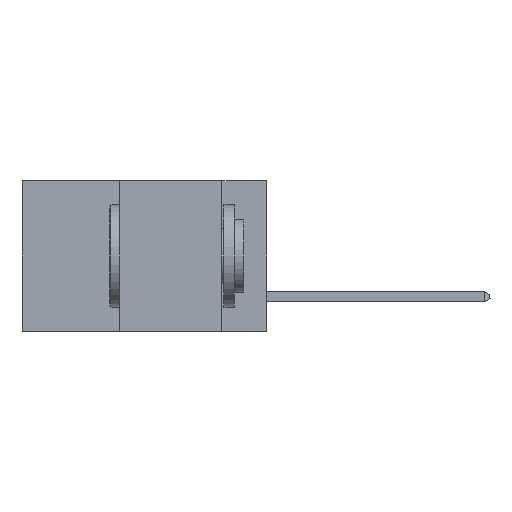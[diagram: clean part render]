
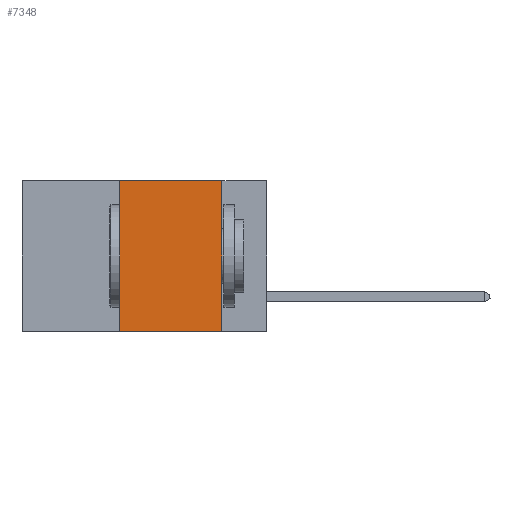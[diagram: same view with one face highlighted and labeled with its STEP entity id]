
A CAD part, left-side view. The second image highlights one B-rep face of the part: STEP entity #7348.
In plain terms, the highlighted planar face has unit normal (-1, 0, 0).
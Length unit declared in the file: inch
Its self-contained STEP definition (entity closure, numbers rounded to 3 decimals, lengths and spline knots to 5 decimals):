
#431 = PLANE ( 'NONE',  #6124 ) ;
#549 = CARTESIAN_POINT ( 'NONE',  ( 0., 0.11, 0. ) ) ;
#1457 = LINE ( 'NONE', #8923, #3112 ) ;
#1663 = EDGE_CURVE ( 'NONE', #2905, #11266, #1457, .T. ) ;
#2905 = VERTEX_POINT ( 'NONE', #17620 ) ;
#3067 = DIRECTION ( 'NONE',  ( 0., -1., 0. ) ) ;
#3112 = VECTOR ( 'NONE', #10930, 39.37008 ) ;
#3294 = ORIENTED_EDGE ( 'NONE', *, *, #11634, .F. ) ;
#3508 = DIRECTION ( 'NONE',  ( 1., 0., 0. ) ) ;
#3814 = VECTOR ( 'NONE', #6072, 39.37008 ) ;
#3959 = ORIENTED_EDGE ( 'NONE', *, *, #1663, .F. ) ;
#4521 = CARTESIAN_POINT ( 'NONE',  ( 0., 0.6, -0.37 ) ) ;
#4826 = DIRECTION ( 'NONE',  ( 0., 0., -1. ) ) ;
#5379 = FACE_OUTER_BOUND ( 'NONE', #9659, .T. ) ;
#5426 = VECTOR ( 'NONE', #3067, 39.37008 ) ;
#6072 = DIRECTION ( 'NONE',  ( 0., 0., -1. ) ) ;
#6124 = AXIS2_PLACEMENT_3D ( 'NONE', #12545, #3508, #4826 ) ;
#6180 = ORIENTED_EDGE ( 'NONE', *, *, #19208, .T. ) ;
#7348 = ADVANCED_FACE ( 'NONE', ( #5379 ), #431, .F. ) ;
#7781 = LINE ( 'NONE', #17904, #3814 ) ;
#8299 = VERTEX_POINT ( 'NONE', #9223 ) ;
#8686 = CARTESIAN_POINT ( 'NONE',  ( 0., 0.11, -0.37 ) ) ;
#8923 = CARTESIAN_POINT ( 'NONE',  ( 0., 0.6, 0. ) ) ;
#9223 = CARTESIAN_POINT ( 'NONE',  ( 0., 0.36, -0.37 ) ) ;
#9659 = EDGE_LOOP ( 'NONE', ( #9702, #3959, #3294, #6180 ) ) ;
#9702 = ORIENTED_EDGE ( 'NONE', *, *, #13621, .F. ) ;
#10371 = VERTEX_POINT ( 'NONE', #8686 ) ;
#10930 = DIRECTION ( 'NONE',  ( 0., -1., 0. ) ) ;
#11266 = VERTEX_POINT ( 'NONE', #549 ) ;
#11634 = EDGE_CURVE ( 'NONE', #8299, #2905, #18638, .T. ) ;
#11795 = DIRECTION ( 'NONE',  ( 0., 0., 1. ) ) ;
#12545 = CARTESIAN_POINT ( 'NONE',  ( 0., 0.6, 0. ) ) ;
#13621 = EDGE_CURVE ( 'NONE', #11266, #10371, #7781, .T. ) ;
#14674 = CARTESIAN_POINT ( 'NONE',  ( 0., 0.36, 0. ) ) ;
#15308 = VECTOR ( 'NONE', #11795, 39.37008 ) ;
#15919 = LINE ( 'NONE', #4521, #5426 ) ;
#17620 = CARTESIAN_POINT ( 'NONE',  ( 0., 0.36, 0. ) ) ;
#17904 = CARTESIAN_POINT ( 'NONE',  ( 0., 0.11, 0. ) ) ;
#18638 = LINE ( 'NONE', #14674, #15308 ) ;
#19208 = EDGE_CURVE ( 'NONE', #8299, #10371, #15919, .T. ) ;
